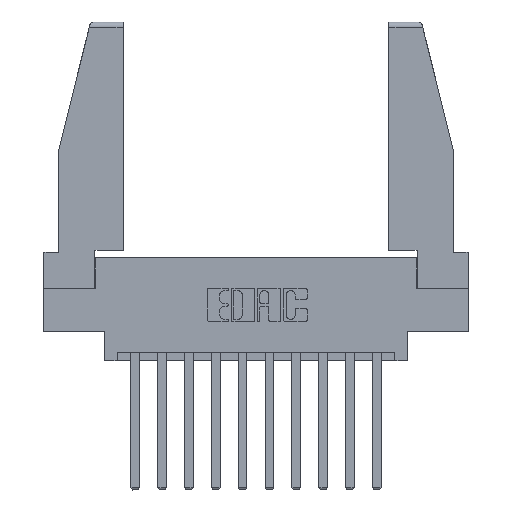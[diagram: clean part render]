
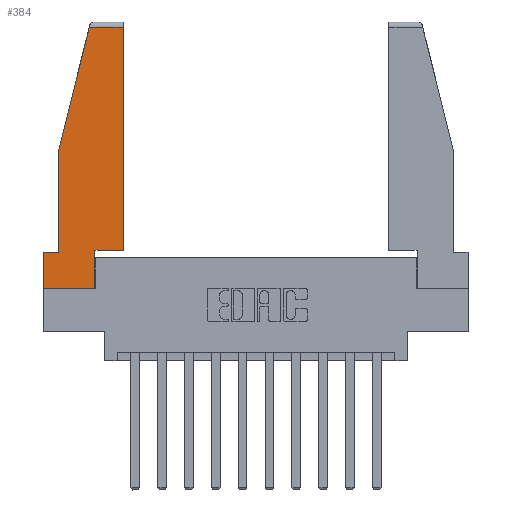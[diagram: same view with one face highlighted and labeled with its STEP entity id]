
A CAD part, top view. The second image highlights one B-rep face of the part: STEP entity #384.
In plain terms, the highlighted planar face has unit normal (0, 0, 1).
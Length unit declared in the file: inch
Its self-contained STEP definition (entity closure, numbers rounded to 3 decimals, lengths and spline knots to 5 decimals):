
#121 = VERTEX_POINT ( 'NONE', #4119 ) ;
#384 = ADVANCED_FACE ( 'NONE', ( #5831 ), #7301, .T. ) ;
#592 = ORIENTED_EDGE ( 'NONE', *, *, #7373, .T. ) ;
#611 = LINE ( 'NONE', #14275, #3545 ) ;
#705 = VECTOR ( 'NONE', #9884, 39.37008 ) ;
#1647 = VECTOR ( 'NONE', #6432, 39.37008 ) ;
#1716 = DIRECTION ( 'NONE',  ( 0., 0., 1. ) ) ;
#2207 = DIRECTION ( 'NONE',  ( 0., 1., 0. ) ) ;
#2345 = LINE ( 'NONE', #4289, #1647 ) ;
#2364 = CARTESIAN_POINT ( 'NONE',  ( 0.297, 0., 0. ) ) ;
#2898 = ORIENTED_EDGE ( 'NONE', *, *, #10301, .T. ) ;
#3124 = VERTEX_POINT ( 'NONE', #2364 ) ;
#3174 = EDGE_CURVE ( 'NONE', #6449, #13575, #611, .T. ) ;
#3217 = LINE ( 'NONE', #9605, #9953 ) ;
#3375 = CARTESIAN_POINT ( 'NONE',  ( 0., 1.52, 0. ) ) ;
#3489 = EDGE_CURVE ( 'NONE', #12040, #6389, #2345, .T. ) ;
#3545 = VECTOR ( 'NONE', #2207, 39.37008 ) ;
#3585 = CARTESIAN_POINT ( 'NONE',  ( 0.271, 1.55, 0. ) ) ;
#3931 = VECTOR ( 'NONE', #4081, 39.37008 ) ;
#3999 = DIRECTION ( 'NONE',  ( 1., 0., 0. ) ) ;
#4081 = DIRECTION ( 'NONE',  ( 0., -1., 0. ) ) ;
#4119 = CARTESIAN_POINT ( 'NONE',  ( 0.297, 0.223, 0. ) ) ;
#4289 = CARTESIAN_POINT ( 'NONE',  ( 0., 0.21, 0. ) ) ;
#4414 = CARTESIAN_POINT ( 'NONE',  ( 0.297, 0., 0. ) ) ;
#4814 = VECTOR ( 'NONE', #6691, 39.37008 ) ;
#5414 = DIRECTION ( 'NONE',  ( 0., -1., 0. ) ) ;
#5573 = LINE ( 'NONE', #6402, #14064 ) ;
#5582 = CARTESIAN_POINT ( 'NONE',  ( 0.086, 0.21, 0. ) ) ;
#5831 = FACE_OUTER_BOUND ( 'NONE', #10166, .T. ) ;
#5868 = LINE ( 'NONE', #4414, #11430 ) ;
#5960 = ORIENTED_EDGE ( 'NONE', *, *, #11780, .T. ) ;
#6238 = ORIENTED_EDGE ( 'NONE', *, *, #13402, .T. ) ;
#6389 = VERTEX_POINT ( 'NONE', #13416 ) ;
#6402 = CARTESIAN_POINT ( 'NONE',  ( 0., 0.21, 0. ) ) ;
#6432 = DIRECTION ( 'NONE',  ( -1., 0., 0. ) ) ;
#6449 = VERTEX_POINT ( 'NONE', #11312 ) ;
#6606 = ORIENTED_EDGE ( 'NONE', *, *, #3174, .T. ) ;
#6612 = ORIENTED_EDGE ( 'NONE', *, *, #13361, .T. ) ;
#6677 = ORIENTED_EDGE ( 'NONE', *, *, #3489, .T. ) ;
#6691 = DIRECTION ( 'NONE',  ( 1., 0., 0. ) ) ;
#7301 = PLANE ( 'NONE',  #11484 ) ;
#7373 = EDGE_CURVE ( 'NONE', #6389, #9694, #5573, .T. ) ;
#8320 = ORIENTED_EDGE ( 'NONE', *, *, #9104, .T. ) ;
#8345 = VERTEX_POINT ( 'NONE', #9637 ) ;
#8458 = ORIENTED_EDGE ( 'NONE', *, *, #10042, .T. ) ;
#8594 = LINE ( 'NONE', #11885, #3931 ) ;
#9104 = EDGE_CURVE ( 'NONE', #3124, #121, #5868, .T. ) ;
#9312 = CARTESIAN_POINT ( 'NONE',  ( 0., 0., 0. ) ) ;
#9605 = CARTESIAN_POINT ( 'NONE',  ( 0., 0., 0. ) ) ;
#9612 = VERTEX_POINT ( 'NONE', #13149 ) ;
#9637 = CARTESIAN_POINT ( 'NONE',  ( 0.2636, 1.52, 0. ) ) ;
#9694 = VERTEX_POINT ( 'NONE', #11535 ) ;
#9884 = DIRECTION ( 'NONE',  ( -0.239, -0.971, 0. ) ) ;
#9953 = VECTOR ( 'NONE', #3999, 39.37008 ) ;
#9982 = CARTESIAN_POINT ( 'NONE',  ( 0.297, 0.223, 0. ) ) ;
#10042 = EDGE_CURVE ( 'NONE', #9612, #12040, #8594, .T. ) ;
#10166 = EDGE_LOOP ( 'NONE', ( #6606, #2898, #6238, #8458, #6677, #592, #5960, #8320, #6612 ) ) ;
#10301 = EDGE_CURVE ( 'NONE', #13575, #8345, #11402, .T. ) ;
#10572 = DIRECTION ( 'NONE',  ( 1., 0., 0. ) ) ;
#10890 = DIRECTION ( 'NONE',  ( -1., 0., 0. ) ) ;
#11312 = CARTESIAN_POINT ( 'NONE',  ( 0.461, 0.223, 0. ) ) ;
#11402 = LINE ( 'NONE', #3375, #12431 ) ;
#11430 = VECTOR ( 'NONE', #12171, 39.37008 ) ;
#11484 = AXIS2_PLACEMENT_3D ( 'NONE', #9312, #1716, #10572 ) ;
#11535 = CARTESIAN_POINT ( 'NONE',  ( 0., 0., 0. ) ) ;
#11761 = LINE ( 'NONE', #9982, #4814 ) ;
#11780 = EDGE_CURVE ( 'NONE', #9694, #3124, #3217, .T. ) ;
#11885 = CARTESIAN_POINT ( 'NONE',  ( 0.086, 0.8, 0. ) ) ;
#12040 = VERTEX_POINT ( 'NONE', #5582 ) ;
#12171 = DIRECTION ( 'NONE',  ( 0., 1., 0. ) ) ;
#12431 = VECTOR ( 'NONE', #10890, 39.37008 ) ;
#12620 = LINE ( 'NONE', #3585, #705 ) ;
#13149 = CARTESIAN_POINT ( 'NONE',  ( 0.086, 0.8, 0. ) ) ;
#13156 = CARTESIAN_POINT ( 'NONE',  ( 0.461, 1.52, 0. ) ) ;
#13361 = EDGE_CURVE ( 'NONE', #121, #6449, #11761, .T. ) ;
#13402 = EDGE_CURVE ( 'NONE', #8345, #9612, #12620, .T. ) ;
#13416 = CARTESIAN_POINT ( 'NONE',  ( 0., 0.21, 0. ) ) ;
#13575 = VERTEX_POINT ( 'NONE', #13156 ) ;
#14064 = VECTOR ( 'NONE', #5414, 39.37008 ) ;
#14275 = CARTESIAN_POINT ( 'NONE',  ( 0.461, 0.223, 0. ) ) ;
